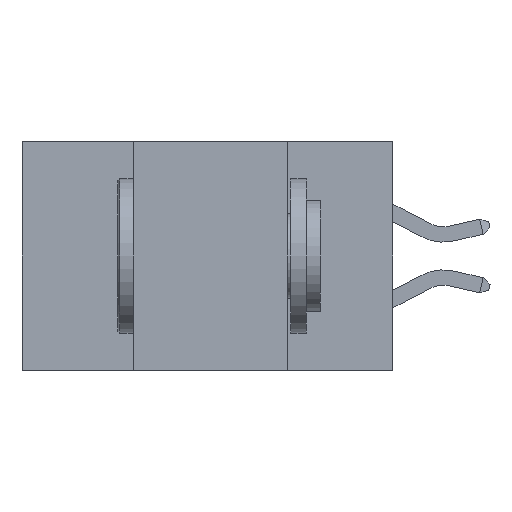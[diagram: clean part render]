
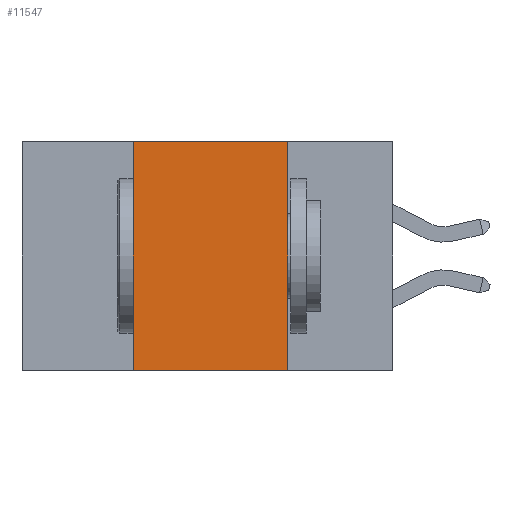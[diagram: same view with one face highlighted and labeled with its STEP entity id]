
A CAD part, left-side view. The second image highlights one B-rep face of the part: STEP entity #11547.
In plain terms, the highlighted planar face has unit normal (-1, 0, 0).
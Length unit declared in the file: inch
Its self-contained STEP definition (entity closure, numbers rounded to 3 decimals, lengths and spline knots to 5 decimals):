
#44 = DIRECTION ( 'NONE',  ( 0., 0., -1. ) ) ;
#315 = AXIS2_PLACEMENT_3D ( 'NONE', #2755, #12730, #2696 ) ;
#457 = EDGE_CURVE ( 'NONE', #12223, #14935, #8989, .T. ) ;
#484 = DIRECTION ( 'NONE',  ( 0., -1., 0. ) ) ;
#975 = EDGE_CURVE ( 'NONE', #7776, #12223, #9170, .T. ) ;
#2696 = DIRECTION ( 'NONE',  ( 0., 0., -1. ) ) ;
#2755 = CARTESIAN_POINT ( 'NONE',  ( 0., 0.6, 0. ) ) ;
#3011 = VECTOR ( 'NONE', #44, 39.37008 ) ;
#4004 = EDGE_CURVE ( 'NONE', #7776, #10270, #10832, .T. ) ;
#4253 = VECTOR ( 'NONE', #484, 39.37008 ) ;
#4803 = EDGE_LOOP ( 'NONE', ( #10023, #5940, #9889, #6891 ) ) ;
#5023 = VECTOR ( 'NONE', #8006, 39.37008 ) ;
#5416 = PLANE ( 'NONE',  #315 ) ;
#5940 = ORIENTED_EDGE ( 'NONE', *, *, #457, .F. ) ;
#6420 = CARTESIAN_POINT ( 'NONE',  ( 0., 0.17, -0.37 ) ) ;
#6891 = ORIENTED_EDGE ( 'NONE', *, *, #4004, .T. ) ;
#7354 = EDGE_CURVE ( 'NONE', #14935, #10270, #9738, .T. ) ;
#7776 = VERTEX_POINT ( 'NONE', #16363 ) ;
#8006 = DIRECTION ( 'NONE',  ( 0., 0., 1. ) ) ;
#8989 = LINE ( 'NONE', #10677, #9957 ) ;
#9170 = LINE ( 'NONE', #15564, #5023 ) ;
#9738 = LINE ( 'NONE', #10032, #3011 ) ;
#9889 = ORIENTED_EDGE ( 'NONE', *, *, #975, .F. ) ;
#9957 = VECTOR ( 'NONE', #16073, 39.37008 ) ;
#9972 = FACE_OUTER_BOUND ( 'NONE', #4803, .T. ) ;
#10023 = ORIENTED_EDGE ( 'NONE', *, *, #7354, .F. ) ;
#10032 = CARTESIAN_POINT ( 'NONE',  ( 0., 0.17, 0. ) ) ;
#10270 = VERTEX_POINT ( 'NONE', #6420 ) ;
#10552 = CARTESIAN_POINT ( 'NONE',  ( 0., 0.6, -0.37 ) ) ;
#10677 = CARTESIAN_POINT ( 'NONE',  ( 0., 0.6, 0. ) ) ;
#10832 = LINE ( 'NONE', #10552, #4253 ) ;
#11547 = ADVANCED_FACE ( 'NONE', ( #9972 ), #5416, .F. ) ;
#12223 = VERTEX_POINT ( 'NONE', #13312 ) ;
#12730 = DIRECTION ( 'NONE',  ( 1., 0., 0. ) ) ;
#13312 = CARTESIAN_POINT ( 'NONE',  ( 0., 0.42, 0. ) ) ;
#14935 = VERTEX_POINT ( 'NONE', #15782 ) ;
#15564 = CARTESIAN_POINT ( 'NONE',  ( 0., 0.42, 0. ) ) ;
#15782 = CARTESIAN_POINT ( 'NONE',  ( 0., 0.17, 0. ) ) ;
#16073 = DIRECTION ( 'NONE',  ( 0., -1., 0. ) ) ;
#16363 = CARTESIAN_POINT ( 'NONE',  ( 0., 0.42, -0.37 ) ) ;
